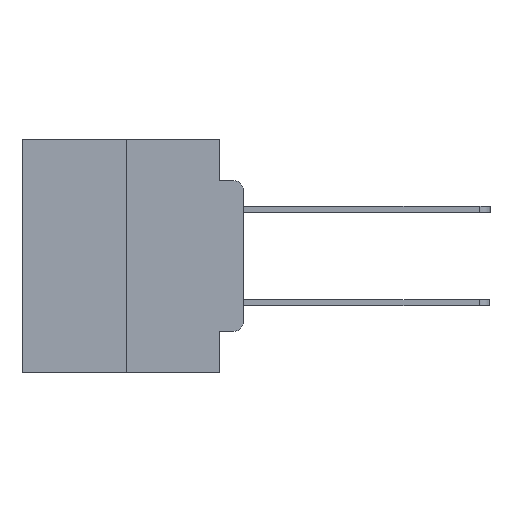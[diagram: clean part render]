
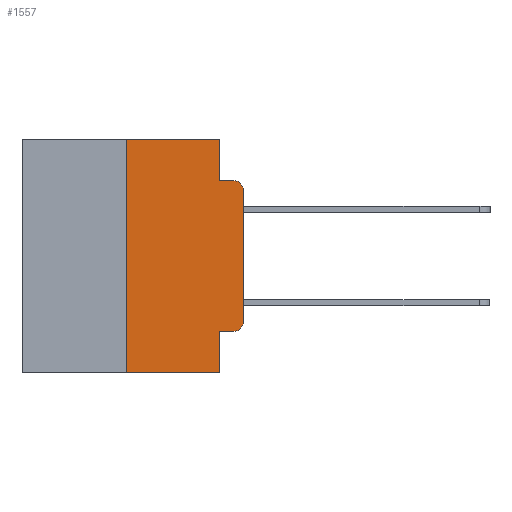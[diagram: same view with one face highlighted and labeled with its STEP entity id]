
A CAD part, left-side view. The second image highlights one B-rep face of the part: STEP entity #1557.
In plain terms, the highlighted planar face has unit normal (-1, 0, 0).
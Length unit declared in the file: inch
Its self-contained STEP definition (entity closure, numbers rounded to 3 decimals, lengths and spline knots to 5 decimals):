
#868 = VERTEX_POINT ( 'NONE', #22249 ) ;
#1099 = PLANE ( 'NONE',  #10033 ) ;
#1177 = CARTESIAN_POINT ( 'NONE',  ( 0., 0.25, -0.5 ) ) ;
#1422 = CARTESIAN_POINT ( 'NONE',  ( 0., 0.02, -0.1085 ) ) ;
#1557 = ADVANCED_FACE ( 'NONE', ( #23083 ), #1099, .F. ) ;
#1735 = CARTESIAN_POINT ( 'NONE',  ( 0., 0.051, 0. ) ) ;
#2226 = VERTEX_POINT ( 'NONE', #8138 ) ;
#2341 = AXIS2_PLACEMENT_3D ( 'NONE', #6647, #21421, #8818 ) ;
#2425 = EDGE_CURVE ( 'NONE', #7491, #3850, #3171, .T. ) ;
#2678 = CIRCLE ( 'NONE', #2341, 0.02 ) ;
#3171 = LINE ( 'NONE', #19302, #19514 ) ;
#3311 = CARTESIAN_POINT ( 'NONE',  ( 0., 0.473, 0. ) ) ;
#3634 = DIRECTION ( 'NONE',  ( 0., 0., -1. ) ) ;
#3722 = ORIENTED_EDGE ( 'NONE', *, *, #20117, .T. ) ;
#3850 = VERTEX_POINT ( 'NONE', #8284 ) ;
#4678 = EDGE_CURVE ( 'NONE', #11984, #868, #23603, .T. ) ;
#4710 = ORIENTED_EDGE ( 'NONE', *, *, #2425, .F. ) ;
#4714 = LINE ( 'NONE', #25006, #27025 ) ;
#4839 = LINE ( 'NONE', #11581, #21097 ) ;
#4863 = CARTESIAN_POINT ( 'NONE',  ( 0., 0.051, -0.0885 ) ) ;
#5136 = CARTESIAN_POINT ( 'NONE',  ( 0., 0., -0.3915 ) ) ;
#6050 = DIRECTION ( 'NONE',  ( 0., -1., 0. ) ) ;
#6297 = VERTEX_POINT ( 'NONE', #23003 ) ;
#6647 = CARTESIAN_POINT ( 'NONE',  ( 0., 0.02, -0.3915 ) ) ;
#6908 = DIRECTION ( 'NONE',  ( 0., -1., 0. ) ) ;
#7096 = ORIENTED_EDGE ( 'NONE', *, *, #24249, .F. ) ;
#7491 = VERTEX_POINT ( 'NONE', #1177 ) ;
#7683 = DIRECTION ( 'NONE',  ( 0., 0., -1. ) ) ;
#7725 = CARTESIAN_POINT ( 'NONE',  ( 0., 0.051, 0. ) ) ;
#8138 = CARTESIAN_POINT ( 'NONE',  ( 0., 0.051, 0. ) ) ;
#8284 = CARTESIAN_POINT ( 'NONE',  ( 0., 0.25, 0. ) ) ;
#8293 = DIRECTION ( 'NONE',  ( 0., -1., 0. ) ) ;
#8818 = DIRECTION ( 'NONE',  ( 0., 0., -1. ) ) ;
#8985 = EDGE_CURVE ( 'NONE', #15353, #10194, #2678, .T. ) ;
#9683 = VECTOR ( 'NONE', #24962, 39.37008 ) ;
#10000 = VECTOR ( 'NONE', #20128, 39.37008 ) ;
#10033 = AXIS2_PLACEMENT_3D ( 'NONE', #3311, #20335, #7683 ) ;
#10194 = VERTEX_POINT ( 'NONE', #5136 ) ;
#10376 = ORIENTED_EDGE ( 'NONE', *, *, #4678, .F. ) ;
#10387 = CARTESIAN_POINT ( 'NONE',  ( 0., 0.02, -0.4115 ) ) ;
#11136 = EDGE_CURVE ( 'NONE', #2226, #11984, #15341, .T. ) ;
#11206 = CARTESIAN_POINT ( 'NONE',  ( 0., 0.051, -0.0885 ) ) ;
#11581 = CARTESIAN_POINT ( 'NONE',  ( 0., 0., 0. ) ) ;
#11984 = VERTEX_POINT ( 'NONE', #4863 ) ;
#12090 = VERTEX_POINT ( 'NONE', #26174 ) ;
#12546 = VECTOR ( 'NONE', #6908, 39.37008 ) ;
#13386 = ORIENTED_EDGE ( 'NONE', *, *, #18937, .T. ) ;
#13722 = DIRECTION ( 'NONE',  ( 0., 0., 1. ) ) ;
#14520 = EDGE_CURVE ( 'NONE', #24458, #15353, #26387, .T. ) ;
#15341 = LINE ( 'NONE', #1735, #9683 ) ;
#15353 = VERTEX_POINT ( 'NONE', #10387 ) ;
#15663 = LINE ( 'NONE', #26215, #10000 ) ;
#16425 = EDGE_LOOP ( 'NONE', ( #21227, #13386, #10376, #18679, #7096, #4710, #3722, #21401, #18489, #25891 ) ) ;
#16459 = DIRECTION ( 'NONE',  ( -1., 0., 0. ) ) ;
#17080 = AXIS2_PLACEMENT_3D ( 'NONE', #1422, #16459, #3634 ) ;
#18489 = ORIENTED_EDGE ( 'NONE', *, *, #14520, .T. ) ;
#18679 = ORIENTED_EDGE ( 'NONE', *, *, #11136, .F. ) ;
#18771 = CARTESIAN_POINT ( 'NONE',  ( 0., 0.051, -0.4115 ) ) ;
#18937 = EDGE_CURVE ( 'NONE', #6297, #868, #19120, .T. ) ;
#19120 = CIRCLE ( 'NONE', #17080, 0.02 ) ;
#19174 = VECTOR ( 'NONE', #24482, 39.37008 ) ;
#19302 = CARTESIAN_POINT ( 'NONE',  ( 0., 0.25, 0. ) ) ;
#19445 = CARTESIAN_POINT ( 'NONE',  ( 0., 0.051, -0.4115 ) ) ;
#19514 = VECTOR ( 'NONE', #23338, 39.37008 ) ;
#20117 = EDGE_CURVE ( 'NONE', #7491, #12090, #15663, .T. ) ;
#20128 = DIRECTION ( 'NONE',  ( 0., -1., 0. ) ) ;
#20335 = DIRECTION ( 'NONE',  ( 1., 0., 0. ) ) ;
#21097 = VECTOR ( 'NONE', #13722, 39.37008 ) ;
#21117 = LINE ( 'NONE', #7725, #19174 ) ;
#21227 = ORIENTED_EDGE ( 'NONE', *, *, #27162, .T. ) ;
#21401 = ORIENTED_EDGE ( 'NONE', *, *, #21500, .F. ) ;
#21421 = DIRECTION ( 'NONE',  ( -1., 0., 0. ) ) ;
#21500 = EDGE_CURVE ( 'NONE', #24458, #12090, #21117, .T. ) ;
#22249 = CARTESIAN_POINT ( 'NONE',  ( 0., 0.02, -0.0885 ) ) ;
#23003 = CARTESIAN_POINT ( 'NONE',  ( 0., 0., -0.1085 ) ) ;
#23083 = FACE_OUTER_BOUND ( 'NONE', #16425, .T. ) ;
#23338 = DIRECTION ( 'NONE',  ( 0., 0., 1. ) ) ;
#23603 = LINE ( 'NONE', #11206, #12546 ) ;
#24249 = EDGE_CURVE ( 'NONE', #3850, #2226, #4714, .T. ) ;
#24458 = VERTEX_POINT ( 'NONE', #19445 ) ;
#24482 = DIRECTION ( 'NONE',  ( 0., 0., -1. ) ) ;
#24962 = DIRECTION ( 'NONE',  ( 0., 0., -1. ) ) ;
#25006 = CARTESIAN_POINT ( 'NONE',  ( 0., 0.473, 0. ) ) ;
#25758 = VECTOR ( 'NONE', #6050, 39.37008 ) ;
#25891 = ORIENTED_EDGE ( 'NONE', *, *, #8985, .T. ) ;
#26174 = CARTESIAN_POINT ( 'NONE',  ( 0., 0.051, -0.5 ) ) ;
#26215 = CARTESIAN_POINT ( 'NONE',  ( 0., 0.473, -0.5 ) ) ;
#26387 = LINE ( 'NONE', #18771, #25758 ) ;
#27025 = VECTOR ( 'NONE', #8293, 39.37008 ) ;
#27162 = EDGE_CURVE ( 'NONE', #10194, #6297, #4839, .T. ) ;
